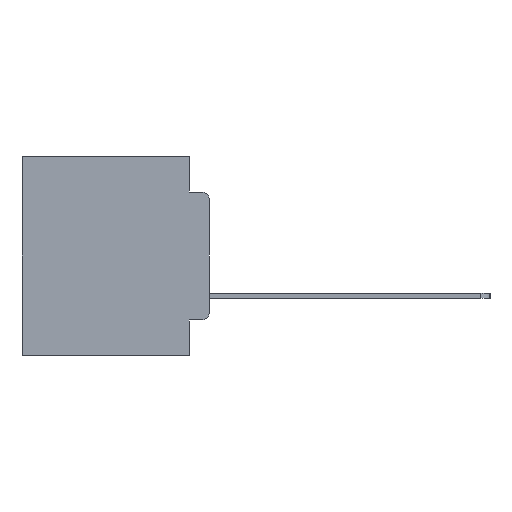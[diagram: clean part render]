
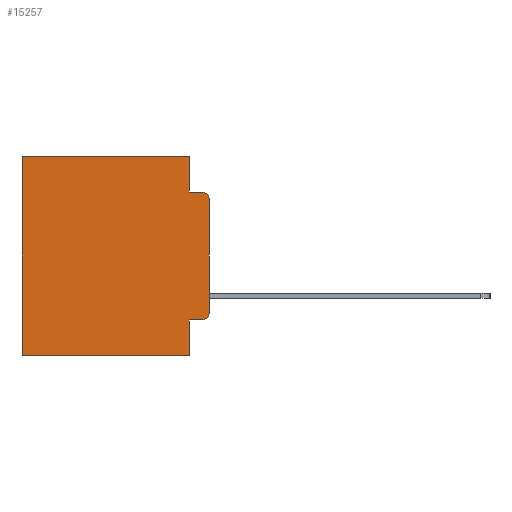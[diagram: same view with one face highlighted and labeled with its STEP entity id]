
A CAD part, left-side view. The second image highlights one B-rep face of the part: STEP entity #15257.
In plain terms, the highlighted planar face has unit normal (-1, 0, 0).
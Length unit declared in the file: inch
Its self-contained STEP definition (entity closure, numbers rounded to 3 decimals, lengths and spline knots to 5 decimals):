
#408 = ORIENTED_EDGE ( 'NONE', *, *, #2794, .F. ) ;
#556 = DIRECTION ( 'NONE',  ( -1., 0., 0. ) ) ;
#1014 = DIRECTION ( 'NONE',  ( 0., 1., 0. ) ) ;
#1351 = CARTESIAN_POINT ( 'NONE',  ( 0.298, 0., -0.3915 ) ) ;
#1439 = EDGE_CURVE ( 'NONE', #17689, #19517, #25220, .T. ) ;
#1699 = LINE ( 'NONE', #5421, #16511 ) ;
#2794 = EDGE_CURVE ( 'NONE', #6212, #3994, #3439, .T. ) ;
#2822 = CARTESIAN_POINT ( 'NONE',  ( 0.298, 0.051, -0.0885 ) ) ;
#3308 = ORIENTED_EDGE ( 'NONE', *, *, #6286, .T. ) ;
#3439 = LINE ( 'NONE', #2822, #13543 ) ;
#3464 = ORIENTED_EDGE ( 'NONE', *, *, #14205, .T. ) ;
#3912 = VECTOR ( 'NONE', #24617, 39.37008 ) ;
#3994 = VERTEX_POINT ( 'NONE', #21730 ) ;
#4064 = ORIENTED_EDGE ( 'NONE', *, *, #19538, .F. ) ;
#4387 = EDGE_CURVE ( 'NONE', #14943, #19517, #7800, .T. ) ;
#4608 = VECTOR ( 'NONE', #20652, 39.37008 ) ;
#4754 = ORIENTED_EDGE ( 'NONE', *, *, #14843, .T. ) ;
#4775 = CARTESIAN_POINT ( 'NONE',  ( 0.298, 0., 0. ) ) ;
#4856 = LINE ( 'NONE', #7790, #20257 ) ;
#4968 = ORIENTED_EDGE ( 'NONE', *, *, #6598, .F. ) ;
#5083 = AXIS2_PLACEMENT_3D ( 'NONE', #7921, #11944, #25796 ) ;
#5421 = CARTESIAN_POINT ( 'NONE',  ( 0.298, 0.051, 0. ) ) ;
#5678 = VERTEX_POINT ( 'NONE', #11754 ) ;
#5736 = AXIS2_PLACEMENT_3D ( 'NONE', #21247, #21762, #22015 ) ;
#6212 = VERTEX_POINT ( 'NONE', #25428 ) ;
#6286 = EDGE_CURVE ( 'NONE', #16321, #14943, #4856, .T. ) ;
#6586 = DIRECTION ( 'NONE',  ( 0., 0., -1. ) ) ;
#6598 = EDGE_CURVE ( 'NONE', #21201, #21818, #13355, .T. ) ;
#7483 = DIRECTION ( 'NONE',  ( 0., 0., -1. ) ) ;
#7790 = CARTESIAN_POINT ( 'NONE',  ( 0.298, 0.051, -0.4115 ) ) ;
#7800 = CIRCLE ( 'NONE', #5736, 0.02 ) ;
#7921 = CARTESIAN_POINT ( 'NONE',  ( 0.298, 0., 0. ) ) ;
#7939 = CARTESIAN_POINT ( 'NONE',  ( 0.298, 0.473, 0. ) ) ;
#8045 = VECTOR ( 'NONE', #1014, 39.37008 ) ;
#8364 = EDGE_CURVE ( 'NONE', #5678, #6212, #8798, .T. ) ;
#8656 = ORIENTED_EDGE ( 'NONE', *, *, #8364, .F. ) ;
#8768 = VECTOR ( 'NONE', #16918, 39.37008 ) ;
#8798 = LINE ( 'NONE', #18617, #14090 ) ;
#8959 = ORIENTED_EDGE ( 'NONE', *, *, #4387, .T. ) ;
#10825 = FACE_OUTER_BOUND ( 'NONE', #15470, .T. ) ;
#11754 = CARTESIAN_POINT ( 'NONE',  ( 0.298, 0.051, 0. ) ) ;
#11944 = DIRECTION ( 'NONE',  ( 1., 0., 0. ) ) ;
#12675 = CARTESIAN_POINT ( 'NONE',  ( 0.298, 0.02, -0.1085 ) ) ;
#13355 = LINE ( 'NONE', #19056, #8045 ) ;
#13543 = VECTOR ( 'NONE', #23805, 39.37008 ) ;
#13812 = CARTESIAN_POINT ( 'NONE',  ( 0.298, 0.051, -0.4115 ) ) ;
#13820 = DIRECTION ( 'NONE',  ( 0., -1., 0. ) ) ;
#14090 = VECTOR ( 'NONE', #6586, 39.37008 ) ;
#14205 = EDGE_CURVE ( 'NONE', #17748, #21818, #19945, .T. ) ;
#14680 = DIRECTION ( 'NONE',  ( 0., 0., -1. ) ) ;
#14843 = EDGE_CURVE ( 'NONE', #17689, #3994, #20217, .T. ) ;
#14943 = VERTEX_POINT ( 'NONE', #22911 ) ;
#15257 = ADVANCED_FACE ( 'NONE', ( #10825 ), #23888, .F. ) ;
#15470 = EDGE_LOOP ( 'NONE', ( #15921, #4754, #408, #8656, #20035, #3464, #4968, #4064, #3308, #8959 ) ) ;
#15921 = ORIENTED_EDGE ( 'NONE', *, *, #1439, .F. ) ;
#16321 = VERTEX_POINT ( 'NONE', #13812 ) ;
#16511 = VECTOR ( 'NONE', #7483, 39.37008 ) ;
#16918 = DIRECTION ( 'NONE',  ( 0., 1., 0. ) ) ;
#17689 = VERTEX_POINT ( 'NONE', #21506 ) ;
#17748 = VERTEX_POINT ( 'NONE', #7939 ) ;
#18617 = CARTESIAN_POINT ( 'NONE',  ( 0.298, 0.051, 0. ) ) ;
#19056 = CARTESIAN_POINT ( 'NONE',  ( 0.298, 0., -0.5 ) ) ;
#19517 = VERTEX_POINT ( 'NONE', #1351 ) ;
#19538 = EDGE_CURVE ( 'NONE', #16321, #21201, #1699, .T. ) ;
#19945 = LINE ( 'NONE', #22695, #3912 ) ;
#20035 = ORIENTED_EDGE ( 'NONE', *, *, #24042, .T. ) ;
#20217 = CIRCLE ( 'NONE', #20911, 0.02 ) ;
#20257 = VECTOR ( 'NONE', #13820, 39.37008 ) ;
#20652 = DIRECTION ( 'NONE',  ( 0., 0., -1. ) ) ;
#20911 = AXIS2_PLACEMENT_3D ( 'NONE', #12675, #556, #14680 ) ;
#20943 = CARTESIAN_POINT ( 'NONE',  ( 0.298, 0.051, -0.5 ) ) ;
#21201 = VERTEX_POINT ( 'NONE', #20943 ) ;
#21247 = CARTESIAN_POINT ( 'NONE',  ( 0.298, 0.02, -0.3915 ) ) ;
#21435 = CARTESIAN_POINT ( 'NONE',  ( 0.298, 0., 0. ) ) ;
#21506 = CARTESIAN_POINT ( 'NONE',  ( 0.298, 0., -0.1085 ) ) ;
#21730 = CARTESIAN_POINT ( 'NONE',  ( 0.298, 0.02, -0.0885 ) ) ;
#21762 = DIRECTION ( 'NONE',  ( -1., 0., 0. ) ) ;
#21818 = VERTEX_POINT ( 'NONE', #23345 ) ;
#22015 = DIRECTION ( 'NONE',  ( 0., 0., -1. ) ) ;
#22695 = CARTESIAN_POINT ( 'NONE',  ( 0.298, 0.473, 0. ) ) ;
#22911 = CARTESIAN_POINT ( 'NONE',  ( 0.298, 0.02, -0.4115 ) ) ;
#23345 = CARTESIAN_POINT ( 'NONE',  ( 0.298, 0.473, -0.5 ) ) ;
#23805 = DIRECTION ( 'NONE',  ( 0., -1., 0. ) ) ;
#23888 = PLANE ( 'NONE',  #5083 ) ;
#24042 = EDGE_CURVE ( 'NONE', #5678, #17748, #24629, .T. ) ;
#24617 = DIRECTION ( 'NONE',  ( 0., 0., -1. ) ) ;
#24629 = LINE ( 'NONE', #4775, #8768 ) ;
#25220 = LINE ( 'NONE', #21435, #4608 ) ;
#25428 = CARTESIAN_POINT ( 'NONE',  ( 0.298, 0.051, -0.0885 ) ) ;
#25796 = DIRECTION ( 'NONE',  ( 0., 0., -1. ) ) ;
